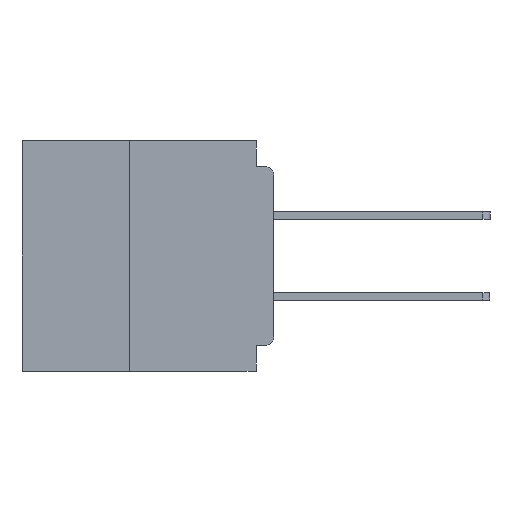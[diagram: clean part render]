
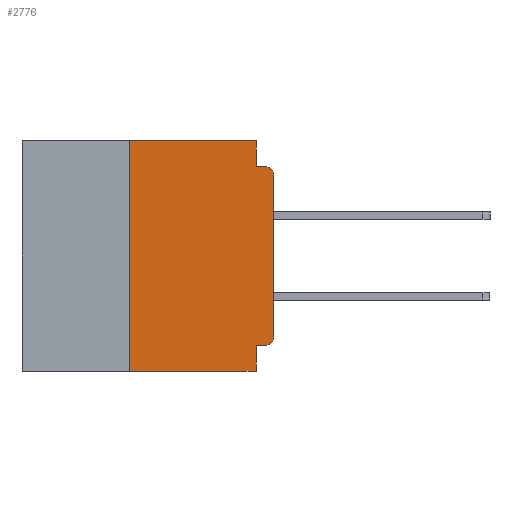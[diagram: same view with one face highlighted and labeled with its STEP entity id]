
A CAD part, left-side view. The second image highlights one B-rep face of the part: STEP entity #2776.
In plain terms, the highlighted planar face has unit normal (-1, 0, 0).
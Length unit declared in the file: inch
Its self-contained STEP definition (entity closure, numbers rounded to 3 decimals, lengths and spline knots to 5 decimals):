
#979 = ORIENTED_EDGE ( 'NONE', *, *, #51627, .F. ) ;
#1219 = AXIS2_PLACEMENT_3D ( 'NONE', #5659, #37808, #10323 ) ;
#1248 = ORIENTED_EDGE ( 'NONE', *, *, #21491, .T. ) ;
#1614 = VECTOR ( 'NONE', #56560, 39.37008 ) ;
#2024 = CARTESIAN_POINT ( 'NONE',  ( 0., 0.015, -0.045 ) ) ;
#2776 = ADVANCED_FACE ( 'NONE', ( #33350 ), #47658, .F. ) ;
#3186 = VECTOR ( 'NONE', #59433, 39.37008 ) ;
#3222 = ORIENTED_EDGE ( 'NONE', *, *, #22383, .F. ) ;
#3823 = CARTESIAN_POINT ( 'NONE',  ( 0., 0.031, 0. ) ) ;
#3847 = CARTESIAN_POINT ( 'NONE',  ( 0., 0.031, -0.4 ) ) ;
#4191 = ORIENTED_EDGE ( 'NONE', *, *, #50965, .F. ) ;
#4198 = EDGE_CURVE ( 'NONE', #53137, #19566, #13717, .T. ) ;
#4471 = ORIENTED_EDGE ( 'NONE', *, *, #44009, .F. ) ;
#5659 = CARTESIAN_POINT ( 'NONE',  ( 0., 0.015, -0.06 ) ) ;
#8471 = DIRECTION ( 'NONE',  ( 0., 1., 0. ) ) ;
#8521 = CARTESIAN_POINT ( 'NONE',  ( 0., 0., -0.06 ) ) ;
#8553 = VERTEX_POINT ( 'NONE', #33626 ) ;
#9371 = CARTESIAN_POINT ( 'NONE',  ( 0., 0.437, 0. ) ) ;
#9534 = CARTESIAN_POINT ( 'NONE',  ( 0., 0.437, -0.4 ) ) ;
#9675 = VECTOR ( 'NONE', #45043, 39.37008 ) ;
#10323 = DIRECTION ( 'NONE',  ( 0., 0., -1. ) ) ;
#10445 = CARTESIAN_POINT ( 'NONE',  ( 0., 0.015, -0.355 ) ) ;
#11122 = LINE ( 'NONE', #9534, #58399 ) ;
#11244 = VERTEX_POINT ( 'NONE', #8521 ) ;
#11371 = EDGE_CURVE ( 'NONE', #31784, #8553, #11122, .T. ) ;
#11484 = EDGE_CURVE ( 'NONE', #11244, #13195, #17563, .T. ) ;
#13097 = CARTESIAN_POINT ( 'NONE',  ( 0., 0., -0.34 ) ) ;
#13195 = VERTEX_POINT ( 'NONE', #2024 ) ;
#13717 = CIRCLE ( 'NONE', #16347, 0.015 ) ;
#13987 = DIRECTION ( 'NONE',  ( 0., -1., 0. ) ) ;
#14107 = LINE ( 'NONE', #36025, #52103 ) ;
#14628 = EDGE_CURVE ( 'NONE', #52754, #8553, #56988, .T. ) ;
#14896 = VERTEX_POINT ( 'NONE', #24011 ) ;
#15347 = LINE ( 'NONE', #29208, #1614 ) ;
#16347 = AXIS2_PLACEMENT_3D ( 'NONE', #36832, #36816, #36757 ) ;
#16473 = DIRECTION ( 'NONE',  ( 0., 0., -1. ) ) ;
#17355 = ORIENTED_EDGE ( 'NONE', *, *, #33751, .F. ) ;
#17563 = CIRCLE ( 'NONE', #1219, 0.015 ) ;
#18303 = CARTESIAN_POINT ( 'NONE',  ( 0., 0.25, -0.4 ) ) ;
#19566 = VERTEX_POINT ( 'NONE', #13097 ) ;
#21491 = EDGE_CURVE ( 'NONE', #19566, #11244, #26256, .T. ) ;
#22383 = EDGE_CURVE ( 'NONE', #27666, #13195, #15347, .T. ) ;
#24011 = CARTESIAN_POINT ( 'NONE',  ( 0., 0.25, 0. ) ) ;
#25556 = LINE ( 'NONE', #59077, #26993 ) ;
#26256 = LINE ( 'NONE', #27499, #3186 ) ;
#26843 = LINE ( 'NONE', #48544, #51172 ) ;
#26875 = CARTESIAN_POINT ( 'NONE',  ( 0., 0.031, -0.045 ) ) ;
#26993 = VECTOR ( 'NONE', #31752, 39.37008 ) ;
#27499 = CARTESIAN_POINT ( 'NONE',  ( 0., 0., 0. ) ) ;
#27666 = VERTEX_POINT ( 'NONE', #26875 ) ;
#29208 = CARTESIAN_POINT ( 'NONE',  ( 0., 0., -0.045 ) ) ;
#31752 = DIRECTION ( 'NONE',  ( 0., 0., 1. ) ) ;
#31784 = VERTEX_POINT ( 'NONE', #18303 ) ;
#31922 = ORIENTED_EDGE ( 'NONE', *, *, #14628, .F. ) ;
#33350 = FACE_OUTER_BOUND ( 'NONE', #50604, .T. ) ;
#33626 = CARTESIAN_POINT ( 'NONE',  ( 0., 0.031, -0.4 ) ) ;
#33751 = EDGE_CURVE ( 'NONE', #14896, #49588, #45910, .T. ) ;
#35021 = CARTESIAN_POINT ( 'NONE',  ( 0., 0.031, -0.355 ) ) ;
#35502 = ORIENTED_EDGE ( 'NONE', *, *, #4198, .T. ) ;
#36025 = CARTESIAN_POINT ( 'NONE',  ( 0., 0., -0.355 ) ) ;
#36757 = DIRECTION ( 'NONE',  ( 0., 0., -1. ) ) ;
#36816 = DIRECTION ( 'NONE',  ( -1., 0., 0. ) ) ;
#36832 = CARTESIAN_POINT ( 'NONE',  ( 0., 0.015, -0.34 ) ) ;
#37808 = DIRECTION ( 'NONE',  ( -1., 0., 0. ) ) ;
#41602 = DIRECTION ( 'NONE',  ( 0., -1., 0. ) ) ;
#44009 = EDGE_CURVE ( 'NONE', #49588, #27666, #26843, .T. ) ;
#44035 = DIRECTION ( 'NONE',  ( 0., 0., -1. ) ) ;
#44455 = VECTOR ( 'NONE', #13987, 39.37008 ) ;
#44616 = DIRECTION ( 'NONE',  ( 1., 0., 0. ) ) ;
#45043 = DIRECTION ( 'NONE',  ( 0., 0., -1. ) ) ;
#45910 = LINE ( 'NONE', #9371, #44455 ) ;
#47658 = PLANE ( 'NONE',  #49708 ) ;
#48544 = CARTESIAN_POINT ( 'NONE',  ( 0., 0.031, 0. ) ) ;
#49588 = VERTEX_POINT ( 'NONE', #3823 ) ;
#49708 = AXIS2_PLACEMENT_3D ( 'NONE', #50580, #44616, #44035 ) ;
#50060 = ORIENTED_EDGE ( 'NONE', *, *, #11484, .T. ) ;
#50580 = CARTESIAN_POINT ( 'NONE',  ( 0., 0.437, 0. ) ) ;
#50604 = EDGE_LOOP ( 'NONE', ( #1248, #50060, #3222, #4471, #17355, #979, #53793, #31922, #4191, #35502 ) ) ;
#50965 = EDGE_CURVE ( 'NONE', #53137, #52754, #14107, .T. ) ;
#51172 = VECTOR ( 'NONE', #16473, 39.37008 ) ;
#51627 = EDGE_CURVE ( 'NONE', #31784, #14896, #25556, .T. ) ;
#52103 = VECTOR ( 'NONE', #8471, 39.37008 ) ;
#52754 = VERTEX_POINT ( 'NONE', #35021 ) ;
#53137 = VERTEX_POINT ( 'NONE', #10445 ) ;
#53793 = ORIENTED_EDGE ( 'NONE', *, *, #11371, .T. ) ;
#56560 = DIRECTION ( 'NONE',  ( 0., -1., 0. ) ) ;
#56988 = LINE ( 'NONE', #3847, #9675 ) ;
#58399 = VECTOR ( 'NONE', #41602, 39.37008 ) ;
#59077 = CARTESIAN_POINT ( 'NONE',  ( 0., 0.25, -0.4 ) ) ;
#59433 = DIRECTION ( 'NONE',  ( 0., 0., 1. ) ) ;
